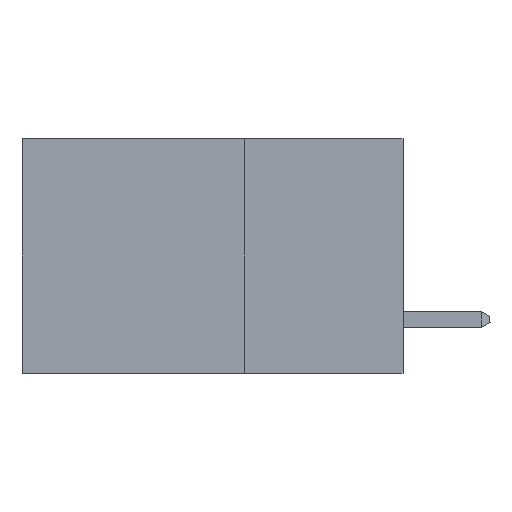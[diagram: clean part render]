
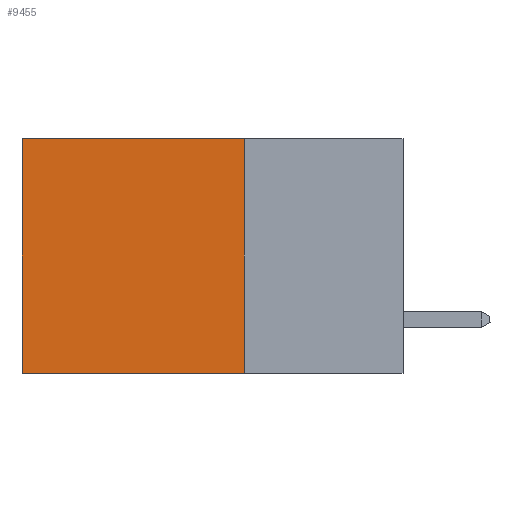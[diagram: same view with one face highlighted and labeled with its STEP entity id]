
A CAD part, left-side view. The second image highlights one B-rep face of the part: STEP entity #9455.
In plain terms, the highlighted planar face has unit normal (-1, 0, 0).
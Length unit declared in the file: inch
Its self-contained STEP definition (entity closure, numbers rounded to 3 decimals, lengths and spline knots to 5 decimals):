
#475 = ORIENTED_EDGE ( 'NONE', *, *, #15719, .T. ) ;
#810 = EDGE_CURVE ( 'NONE', #9385, #5416, #9451, .T. ) ;
#2487 = VECTOR ( 'NONE', #16763, 39.37008 ) ;
#2544 = CARTESIAN_POINT ( 'NONE',  ( 0.2875, 0.25, 0. ) ) ;
#2623 = VECTOR ( 'NONE', #9011, 39.37008 ) ;
#2990 = VECTOR ( 'NONE', #18379, 39.37008 ) ;
#3051 = CARTESIAN_POINT ( 'NONE',  ( 0.2875, 0.25, 0. ) ) ;
#3093 = LINE ( 'NONE', #3051, #2623 ) ;
#3411 = DIRECTION ( 'NONE',  ( 0., 1., 0. ) ) ;
#3656 = EDGE_LOOP ( 'NONE', ( #8896, #10485, #7027, #475 ) ) ;
#5108 = CARTESIAN_POINT ( 'NONE',  ( 0.2875, 0.6, 0. ) ) ;
#5274 = VECTOR ( 'NONE', #3411, 39.37008 ) ;
#5416 = VERTEX_POINT ( 'NONE', #18080 ) ;
#5830 = DIRECTION ( 'NONE',  ( 0., 0., -1. ) ) ;
#7027 = ORIENTED_EDGE ( 'NONE', *, *, #18566, .F. ) ;
#7324 = CARTESIAN_POINT ( 'NONE',  ( 0.2875, 0.25, 0. ) ) ;
#8896 = ORIENTED_EDGE ( 'NONE', *, *, #14137, .T. ) ;
#9011 = DIRECTION ( 'NONE',  ( 0., 1., 0. ) ) ;
#9145 = FACE_OUTER_BOUND ( 'NONE', #3656, .T. ) ;
#9245 = LINE ( 'NONE', #11152, #2487 ) ;
#9316 = LINE ( 'NONE', #13973, #2990 ) ;
#9375 = VERTEX_POINT ( 'NONE', #5108 ) ;
#9385 = VERTEX_POINT ( 'NONE', #18921 ) ;
#9451 = LINE ( 'NONE', #18353, #5274 ) ;
#9455 = ADVANCED_FACE ( 'NONE', ( #9145 ), #14835, .F. ) ;
#10485 = ORIENTED_EDGE ( 'NONE', *, *, #810, .F. ) ;
#11152 = CARTESIAN_POINT ( 'NONE',  ( 0.2875, 0.6, 0. ) ) ;
#13973 = CARTESIAN_POINT ( 'NONE',  ( 0.2875, 0.25, 0. ) ) ;
#14137 = EDGE_CURVE ( 'NONE', #9375, #5416, #9245, .T. ) ;
#14794 = AXIS2_PLACEMENT_3D ( 'NONE', #7324, #16407, #5830 ) ;
#14835 = PLANE ( 'NONE',  #14794 ) ;
#15719 = EDGE_CURVE ( 'NONE', #17299, #9375, #3093, .T. ) ;
#16407 = DIRECTION ( 'NONE',  ( 1., 0., 0. ) ) ;
#16763 = DIRECTION ( 'NONE',  ( 0., 0., -1. ) ) ;
#17299 = VERTEX_POINT ( 'NONE', #2544 ) ;
#18080 = CARTESIAN_POINT ( 'NONE',  ( 0.2875, 0.6, -0.37 ) ) ;
#18353 = CARTESIAN_POINT ( 'NONE',  ( 0.2875, 0.25, -0.37 ) ) ;
#18379 = DIRECTION ( 'NONE',  ( 0., 0., -1. ) ) ;
#18566 = EDGE_CURVE ( 'NONE', #17299, #9385, #9316, .T. ) ;
#18921 = CARTESIAN_POINT ( 'NONE',  ( 0.2875, 0.25, -0.37 ) ) ;
